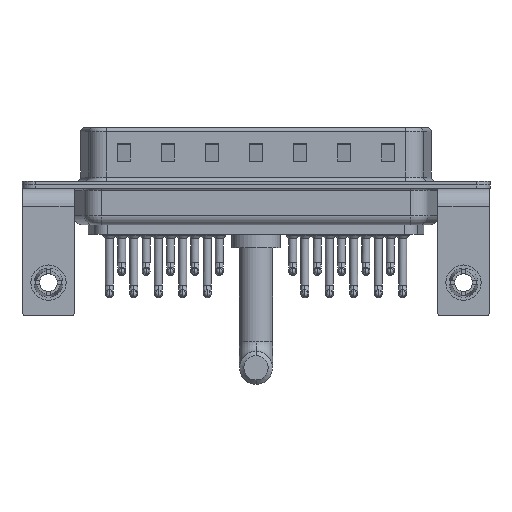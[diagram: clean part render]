
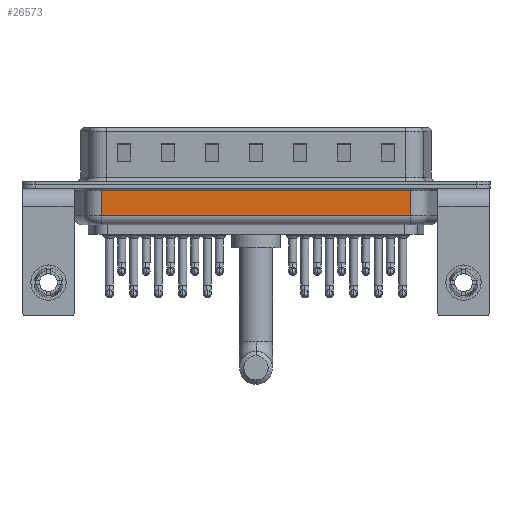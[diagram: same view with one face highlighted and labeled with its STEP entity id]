
A CAD part, front view. The second image highlights one B-rep face of the part: STEP entity #26573.
In plain terms, the highlighted planar face has unit normal (0, -1, 0).
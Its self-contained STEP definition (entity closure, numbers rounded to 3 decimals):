
#245 = DIRECTION ( 'NONE',  ( -1., 0., 0. ) ) ;
#4735 = LINE ( 'NONE', #21846, #5168 ) ;
#5028 = DIRECTION ( 'NONE',  ( 1., 0., 0. ) ) ;
#5168 = VECTOR ( 'NONE', #13509, 1000. ) ;
#5312 = CARTESIAN_POINT ( 'NONE',  ( 6.006, -5.35, -3.5 ) ) ;
#7327 = LINE ( 'NONE', #5312, #23984 ) ;
#7342 = EDGE_CURVE ( 'NONE', #13843, #9450, #4735, .T. ) ;
#7486 = VERTEX_POINT ( 'NONE', #25141 ) ;
#7997 = VERTEX_POINT ( 'NONE', #16060 ) ;
#8129 = CARTESIAN_POINT ( 'NONE',  ( 6.006, -5.35, -0.65 ) ) ;
#8877 = EDGE_LOOP ( 'NONE', ( #28019, #26142, #19575, #11927 ) ) ;
#9450 = VERTEX_POINT ( 'NONE', #8129 ) ;
#11927 = ORIENTED_EDGE ( 'NONE', *, *, #15664, .T. ) ;
#13509 = DIRECTION ( 'NONE',  ( 0., 0., 1. ) ) ;
#13843 = VERTEX_POINT ( 'NONE', #17547 ) ;
#14101 = CARTESIAN_POINT ( 'NONE',  ( 6.006, -5.35, -4.5 ) ) ;
#14172 = EDGE_CURVE ( 'NONE', #13843, #7997, #7327, .T. ) ;
#15664 = EDGE_CURVE ( 'NONE', #7486, #9450, #22102, .T. ) ;
#15992 = PLANE ( 'NONE',  #18483 ) ;
#16060 = CARTESIAN_POINT ( 'NONE',  ( 41.044, -5.35, -3.5 ) ) ;
#16897 = LINE ( 'NONE', #21070, #20272 ) ;
#17547 = CARTESIAN_POINT ( 'NONE',  ( 6.006, -5.35, -3.5 ) ) ;
#18432 = DIRECTION ( 'NONE',  ( 0., 1., 0. ) ) ;
#18483 = AXIS2_PLACEMENT_3D ( 'NONE', #14101, #18432, #27185 ) ;
#19575 = ORIENTED_EDGE ( 'NONE', *, *, #23900, .T. ) ;
#19958 = CARTESIAN_POINT ( 'NONE',  ( 6.006, -5.35, -0.65 ) ) ;
#20272 = VECTOR ( 'NONE', #23070, 1000. ) ;
#21070 = CARTESIAN_POINT ( 'NONE',  ( 41.044, -5.35, -4.5 ) ) ;
#21846 = CARTESIAN_POINT ( 'NONE',  ( 6.006, -5.35, -4.5 ) ) ;
#22102 = LINE ( 'NONE', #19958, #26389 ) ;
#22885 = FACE_OUTER_BOUND ( 'NONE', #8877, .T. ) ;
#23070 = DIRECTION ( 'NONE',  ( 0., 0., 1. ) ) ;
#23900 = EDGE_CURVE ( 'NONE', #7997, #7486, #16897, .T. ) ;
#23984 = VECTOR ( 'NONE', #5028, 1000. ) ;
#25141 = CARTESIAN_POINT ( 'NONE',  ( 41.044, -5.35, -0.65 ) ) ;
#26142 = ORIENTED_EDGE ( 'NONE', *, *, #14172, .T. ) ;
#26389 = VECTOR ( 'NONE', #245, 1000. ) ;
#26573 = ADVANCED_FACE ( 'NONE', ( #22885 ), #15992, .F. ) ;
#27185 = DIRECTION ( 'NONE',  ( 0., 0., 1. ) ) ;
#28019 = ORIENTED_EDGE ( 'NONE', *, *, #7342, .F. ) ;
